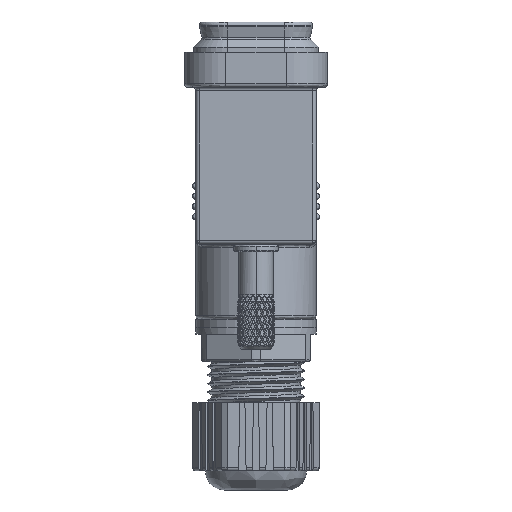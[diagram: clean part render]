
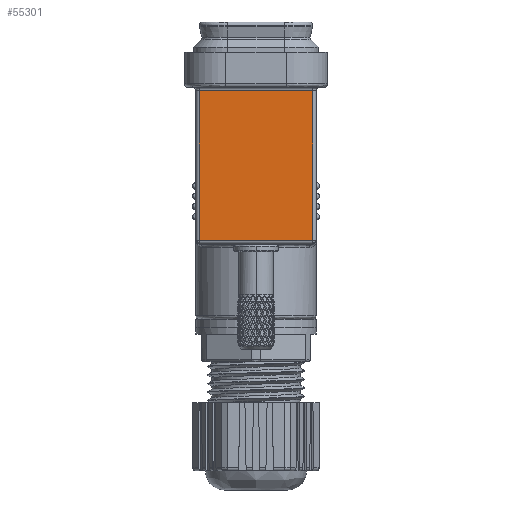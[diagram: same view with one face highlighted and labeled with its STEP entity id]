
A CAD part, front view. The second image highlights one B-rep face of the part: STEP entity #55301.
In plain terms, the highlighted planar face has unit normal (0, -1, 0).
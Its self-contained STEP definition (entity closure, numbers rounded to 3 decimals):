
#485 = ORIENTED_EDGE ( 'NONE', *, *, #77860, .F. ) ;
#2509 = VECTOR ( 'NONE', #38071, 1000. ) ;
#4387 = CARTESIAN_POINT ( 'NONE',  ( 8.3, -27.945, -27.6 ) ) ;
#4706 = AXIS2_PLACEMENT_3D ( 'NONE', #16034, #77234, #65078 ) ;
#12631 = VECTOR ( 'NONE', #50582, 1000. ) ;
#13710 = CARTESIAN_POINT ( 'NONE',  ( -8.3, -27.945, -27.6 ) ) ;
#16034 = CARTESIAN_POINT ( 'NONE',  ( 10.45, -27.945, -32.31 ) ) ;
#21863 = LINE ( 'NONE', #62394, #74597 ) ;
#23641 = DIRECTION ( 'NONE',  ( 1., 0., 0. ) ) ;
#29948 = PLANE ( 'NONE',  #4706 ) ;
#34390 = EDGE_CURVE ( 'NONE', #59326, #52272, #47449, .T. ) ;
#37493 = CARTESIAN_POINT ( 'NONE',  ( 10.45, -27.945, -27.6 ) ) ;
#37942 = VECTOR ( 'NONE', #23641, 1000. ) ;
#38071 = DIRECTION ( 'NONE',  ( 0., 0., 1. ) ) ;
#43497 = ORIENTED_EDGE ( 'NONE', *, *, #82013, .F. ) ;
#45700 = LINE ( 'NONE', #71409, #2509 ) ;
#47449 = LINE ( 'NONE', #37493, #12631 ) ;
#48620 = EDGE_LOOP ( 'NONE', ( #63390, #43497, #79044, #485 ) ) ;
#50582 = DIRECTION ( 'NONE',  ( -1., 0., 0. ) ) ;
#51139 = FACE_OUTER_BOUND ( 'NONE', #48620, .T. ) ;
#52272 = VERTEX_POINT ( 'NONE', #13710 ) ;
#52437 = CARTESIAN_POINT ( 'NONE',  ( 10.45, -27.945, -5.65 ) ) ;
#52873 = LINE ( 'NONE', #52437, #37942 ) ;
#55301 = ADVANCED_FACE ( 'NONE', ( #51139 ), #29948, .F. ) ;
#57089 = CARTESIAN_POINT ( 'NONE',  ( -8.3, -27.945, -5.65 ) ) ;
#58008 = EDGE_CURVE ( 'NONE', #58788, #59900, #52873, .T. ) ;
#58788 = VERTEX_POINT ( 'NONE', #57089 ) ;
#59326 = VERTEX_POINT ( 'NONE', #4387 ) ;
#59900 = VERTEX_POINT ( 'NONE', #74965 ) ;
#62394 = CARTESIAN_POINT ( 'NONE',  ( 8.3, -27.945, -5.024 ) ) ;
#62834 = DIRECTION ( 'NONE',  ( 0., 0., -1. ) ) ;
#63390 = ORIENTED_EDGE ( 'NONE', *, *, #34390, .F. ) ;
#65078 = DIRECTION ( 'NONE',  ( 0., 0., 1. ) ) ;
#71409 = CARTESIAN_POINT ( 'NONE',  ( -8.3, -27.945, -32.31 ) ) ;
#74597 = VECTOR ( 'NONE', #62834, 1000. ) ;
#74965 = CARTESIAN_POINT ( 'NONE',  ( 8.3, -27.945, -5.65 ) ) ;
#77234 = DIRECTION ( 'NONE',  ( 0., 1., 0. ) ) ;
#77860 = EDGE_CURVE ( 'NONE', #52272, #58788, #45700, .T. ) ;
#79044 = ORIENTED_EDGE ( 'NONE', *, *, #58008, .F. ) ;
#82013 = EDGE_CURVE ( 'NONE', #59900, #59326, #21863, .T. ) ;
